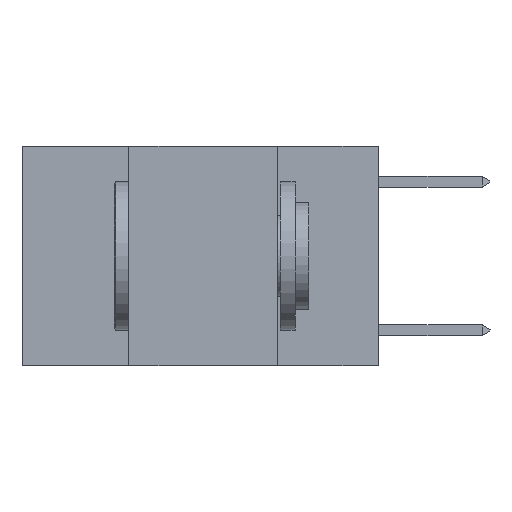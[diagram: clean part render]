
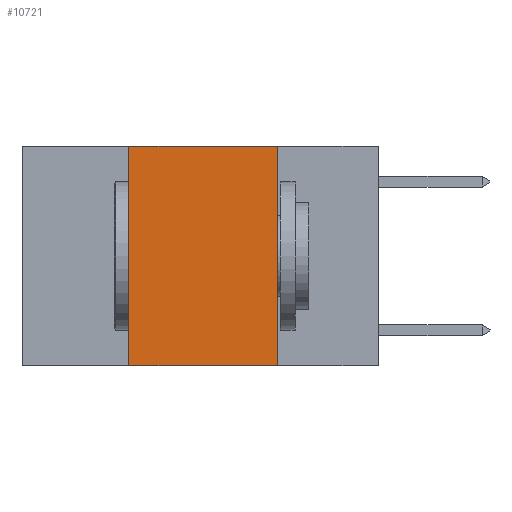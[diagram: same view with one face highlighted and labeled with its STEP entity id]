
A CAD part, left-side view. The second image highlights one B-rep face of the part: STEP entity #10721.
In plain terms, the highlighted planar face has unit normal (-1, 0, 0).
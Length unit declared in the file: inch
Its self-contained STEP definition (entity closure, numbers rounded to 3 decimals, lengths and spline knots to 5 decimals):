
#651 = EDGE_CURVE ( 'NONE', #22338, #11422, #27097, .T. ) ;
#1670 = CARTESIAN_POINT ( 'NONE',  ( 0., 0.6, -0.37 ) ) ;
#3043 = CARTESIAN_POINT ( 'NONE',  ( 0., 0.42, 0. ) ) ;
#3267 = EDGE_CURVE ( 'NONE', #11422, #21430, #13068, .T. ) ;
#3594 = DIRECTION ( 'NONE',  ( 0., -1., 0. ) ) ;
#4093 = CARTESIAN_POINT ( 'NONE',  ( 0., 0.6, 0. ) ) ;
#4579 = EDGE_CURVE ( 'NONE', #6210, #21430, #6609, .T. ) ;
#5638 = CARTESIAN_POINT ( 'NONE',  ( 0., 0.42, 0. ) ) ;
#6210 = VERTEX_POINT ( 'NONE', #21656 ) ;
#6609 = LINE ( 'NONE', #1670, #6642 ) ;
#6642 = VECTOR ( 'NONE', #16870, 39.37008 ) ;
#7318 = EDGE_LOOP ( 'NONE', ( #13915, #13948, #14919, #14937 ) ) ;
#8307 = PLANE ( 'NONE',  #11080 ) ;
#8471 = CARTESIAN_POINT ( 'NONE',  ( 0., 0.17, 0. ) ) ;
#10337 = LINE ( 'NONE', #5638, #21646 ) ;
#10721 = ADVANCED_FACE ( 'NONE', ( #11544 ), #8307, .F. ) ;
#11080 = AXIS2_PLACEMENT_3D ( 'NONE', #27292, #27392, #14811 ) ;
#11422 = VERTEX_POINT ( 'NONE', #8471 ) ;
#11544 = FACE_OUTER_BOUND ( 'NONE', #7318, .T. ) ;
#13014 = VECTOR ( 'NONE', #22645, 39.37008 ) ;
#13068 = LINE ( 'NONE', #18430, #13014 ) ;
#13915 = ORIENTED_EDGE ( 'NONE', *, *, #3267, .F. ) ;
#13948 = ORIENTED_EDGE ( 'NONE', *, *, #651, .F. ) ;
#14811 = DIRECTION ( 'NONE',  ( 0., 0., -1. ) ) ;
#14919 = ORIENTED_EDGE ( 'NONE', *, *, #22467, .F. ) ;
#14937 = ORIENTED_EDGE ( 'NONE', *, *, #4579, .T. ) ;
#16870 = DIRECTION ( 'NONE',  ( 0., -1., 0. ) ) ;
#18430 = CARTESIAN_POINT ( 'NONE',  ( 0., 0.17, 0. ) ) ;
#21430 = VERTEX_POINT ( 'NONE', #23681 ) ;
#21646 = VECTOR ( 'NONE', #22611, 39.37008 ) ;
#21656 = CARTESIAN_POINT ( 'NONE',  ( 0., 0.42, -0.37 ) ) ;
#22338 = VERTEX_POINT ( 'NONE', #3043 ) ;
#22467 = EDGE_CURVE ( 'NONE', #6210, #22338, #10337, .T. ) ;
#22611 = DIRECTION ( 'NONE',  ( 0., 0., 1. ) ) ;
#22645 = DIRECTION ( 'NONE',  ( 0., 0., -1. ) ) ;
#23681 = CARTESIAN_POINT ( 'NONE',  ( 0., 0.17, -0.37 ) ) ;
#27004 = VECTOR ( 'NONE', #3594, 39.37008 ) ;
#27097 = LINE ( 'NONE', #4093, #27004 ) ;
#27292 = CARTESIAN_POINT ( 'NONE',  ( 0., 0.6, 0. ) ) ;
#27392 = DIRECTION ( 'NONE',  ( 1., 0., 0. ) ) ;
